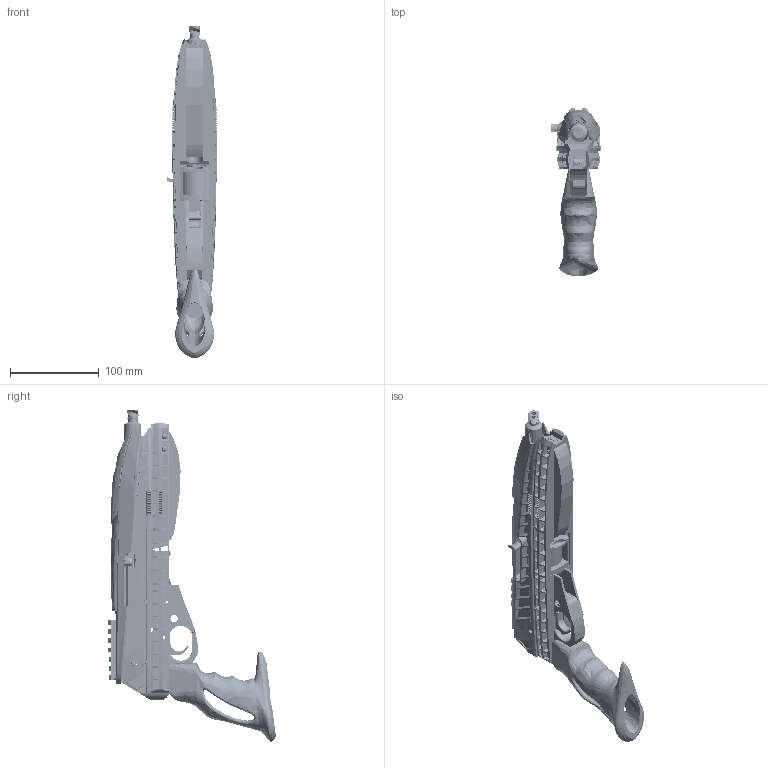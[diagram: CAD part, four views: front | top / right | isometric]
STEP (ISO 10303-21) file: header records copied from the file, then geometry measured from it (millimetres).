
FILE_DESCRIPTION (( 'STEP AP214' ), '1' );
FILE_NAME ('Romulan Charger .22cal v0.5.STEP', '2020-10-11T02:08:43', ( '' ), ( '' ), 'SwSTEP 2.0', 'SolidWorks 2020', '' );
FILE_SCHEMA (( 'AUTOMOTIVE_DESIGN' ));
Length unit declared in the file: inch
Products named in the file (30): Bolt pin bushing; Romulan Charger FCG Housing v0.5; 10-22 Hammer Bushing; 10-22 Hammer; M3 x 8mm Button head 92095A181_92095A181; 10-22 bolt (battlesthecrab); 10-22 receiverpins; Romulan Charger Grip; Romulan Charger forend v0.5; Romulan Charger end plug blank; Ruger 10-22 10 round magazine; Romulan Charger .22cal v0.5; Romulan Charger Receiver v0.5; 8-32x.875 SHCS 92196A198_92196A198; 10-22 Sear; Romulan Charger FCG; 10-22 barrel clamp; Buffer Pin Romulan; Insert 8-32 long 93365A142_93365A142; Bolt Charging handle; 12-24 x 0.5 SHCS 91864A051_91864A051; M3x6mm 91294A126 FLAT-HEAD SOCKET CAP SCREW_91294A126; 10-22 Trigger; Romulan Charger rail; Bolt return pin; Bolt and Handle; 8-32x0.5in SHCS 92196A194_92196A194; Romulan Charger 10-22 barrel 6 inch; 10-22 bolt return spring 96565K370_96565K37
Assembly tree (38 placements, depth 4):
  Romulan Charger .22cal v0.5
    Romulan Charger Receiver v0.5
    Bolt and Handle
      10-22 bolt (battlesthecrab)
      Bolt Charging handle
        Bolt return pin
        10-22 bolt return spring 96565K370_96565K37
        Bolt pin bushing
        Bolt Charging handle
    Romulan Charger FCG
      Romulan Charger FCG Housing v0.5
      10-22 Trigger
      10-22 Sear
      10-22 Hammer
      10-22 Hammer Bushing  x2
    10-22 receiverpins  x2
    Ruger 10-22 10 round magazine
    Romulan Charger 10-22 barrel 6 inch
    Romulan Charger forend v0.5
    Insert 8-32 long 93365A142_93365A142  x2
    8-32x.875 SHCS 92196A198_92196A198
    Romulan Charger Grip
    Buffer Pin Romulan
    Romulan Charger rail
    M3x6mm 91294A126 FLAT-HEAD SOCKET CAP SCREW_91294A126  x3
    8-32x0.5in SHCS 92196A194_92196A194
    10-22 barrel clamp
    12-24 x 0.5 SHCS 91864A051_91864A051  x2
    Romulan Charger end plug blank
    M3 x 8mm Button head 92095A181_92095A181  x4
Bounding box: 57.23 x 189.49 x 374.75 mm (x, y, z)
Volume: 563573.3 mm3; surface area: 273776.5 mm2
Topology: 35 solids, 40 shells, 4646 faces, 12908 edges, 8346 vertices
Faces by surface type: plane 1976, cylinder 1493, bspline 799, cone 312, torus 54, sphere 12
Entity records: 212337 total; most frequent: CARTESIAN_POINT 121350, ORIENTED_EDGE 21900, DIRECTION 14461, EDGE_CURVE 10951, VERTEX_POINT 7092, LINE 5079, VECTOR 5079, AXIS2_PLACEMENT_3D 4691
